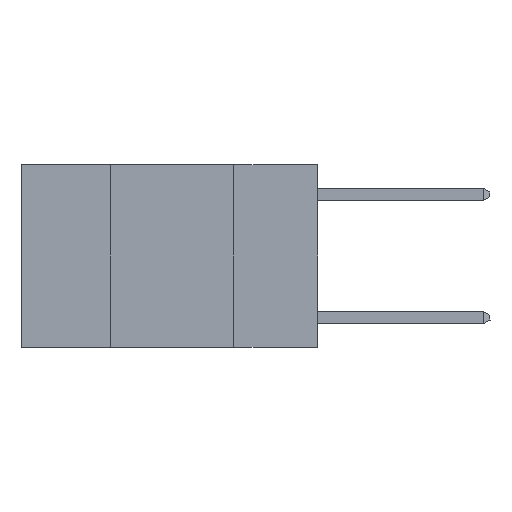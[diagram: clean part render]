
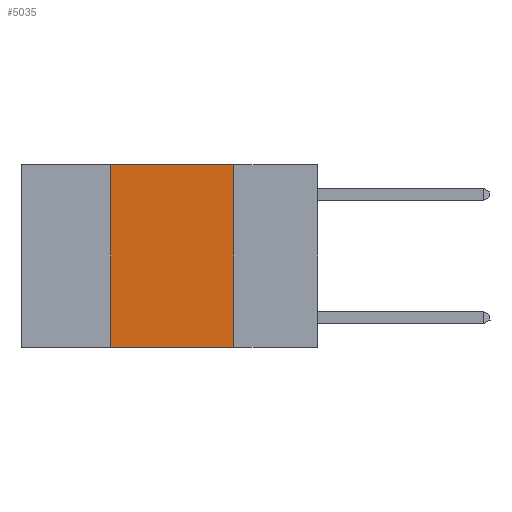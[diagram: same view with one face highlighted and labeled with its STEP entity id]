
A CAD part, left-side view. The second image highlights one B-rep face of the part: STEP entity #5035.
In plain terms, the highlighted planar face has unit normal (-1, 0, 0).
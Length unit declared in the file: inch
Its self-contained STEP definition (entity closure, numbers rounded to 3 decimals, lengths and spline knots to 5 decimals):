
#926 = AXIS2_PLACEMENT_3D ( 'NONE', #8251, #12618, #6142 ) ;
#1227 = VERTEX_POINT ( 'NONE', #10402 ) ;
#1531 = VECTOR ( 'NONE', #8208, 39.37008 ) ;
#1533 = EDGE_CURVE ( 'NONE', #9208, #1227, #2684, .T. ) ;
#2016 = ORIENTED_EDGE ( 'NONE', *, *, #14169, .F. ) ;
#2370 = ORIENTED_EDGE ( 'NONE', *, *, #1533, .F. ) ;
#2607 = FACE_OUTER_BOUND ( 'NONE', #3376, .T. ) ;
#2684 = LINE ( 'NONE', #13278, #13927 ) ;
#2722 = ORIENTED_EDGE ( 'NONE', *, *, #8698, .T. ) ;
#3376 = EDGE_LOOP ( 'NONE', ( #13298, #2016, #2370, #2722 ) ) ;
#3467 = CARTESIAN_POINT ( 'NONE',  ( 0., 0.17, 0. ) ) ;
#3501 = EDGE_CURVE ( 'NONE', #5187, #9943, #7788, .T. ) ;
#3948 = CARTESIAN_POINT ( 'NONE',  ( 0., 0.17, -0.37 ) ) ;
#4521 = LINE ( 'NONE', #4960, #1531 ) ;
#4960 = CARTESIAN_POINT ( 'NONE',  ( 0., 0.6, -0.37 ) ) ;
#5035 = ADVANCED_FACE ( 'NONE', ( #2607 ), #9368, .F. ) ;
#5187 = VERTEX_POINT ( 'NONE', #11751 ) ;
#5742 = LINE ( 'NONE', #10370, #11484 ) ;
#6142 = DIRECTION ( 'NONE',  ( 0., 0., -1. ) ) ;
#7788 = LINE ( 'NONE', #3467, #13206 ) ;
#7881 = DIRECTION ( 'NONE',  ( 0., 0., 1. ) ) ;
#8049 = CARTESIAN_POINT ( 'NONE',  ( 0., 0.42, -0.37 ) ) ;
#8208 = DIRECTION ( 'NONE',  ( 0., -1., 0. ) ) ;
#8251 = CARTESIAN_POINT ( 'NONE',  ( 0., 0.6, 0. ) ) ;
#8698 = EDGE_CURVE ( 'NONE', #9208, #9943, #4521, .T. ) ;
#9208 = VERTEX_POINT ( 'NONE', #8049 ) ;
#9368 = PLANE ( 'NONE',  #926 ) ;
#9943 = VERTEX_POINT ( 'NONE', #3948 ) ;
#10370 = CARTESIAN_POINT ( 'NONE',  ( 0., 0.6, 0. ) ) ;
#10402 = CARTESIAN_POINT ( 'NONE',  ( 0., 0.42, 0. ) ) ;
#11484 = VECTOR ( 'NONE', #13624, 39.37008 ) ;
#11751 = CARTESIAN_POINT ( 'NONE',  ( 0., 0.17, 0. ) ) ;
#12168 = DIRECTION ( 'NONE',  ( 0., 0., -1. ) ) ;
#12618 = DIRECTION ( 'NONE',  ( 1., 0., 0. ) ) ;
#13206 = VECTOR ( 'NONE', #12168, 39.37008 ) ;
#13278 = CARTESIAN_POINT ( 'NONE',  ( 0., 0.42, 0. ) ) ;
#13298 = ORIENTED_EDGE ( 'NONE', *, *, #3501, .F. ) ;
#13624 = DIRECTION ( 'NONE',  ( 0., -1., 0. ) ) ;
#13927 = VECTOR ( 'NONE', #7881, 39.37008 ) ;
#14169 = EDGE_CURVE ( 'NONE', #1227, #5187, #5742, .T. ) ;
